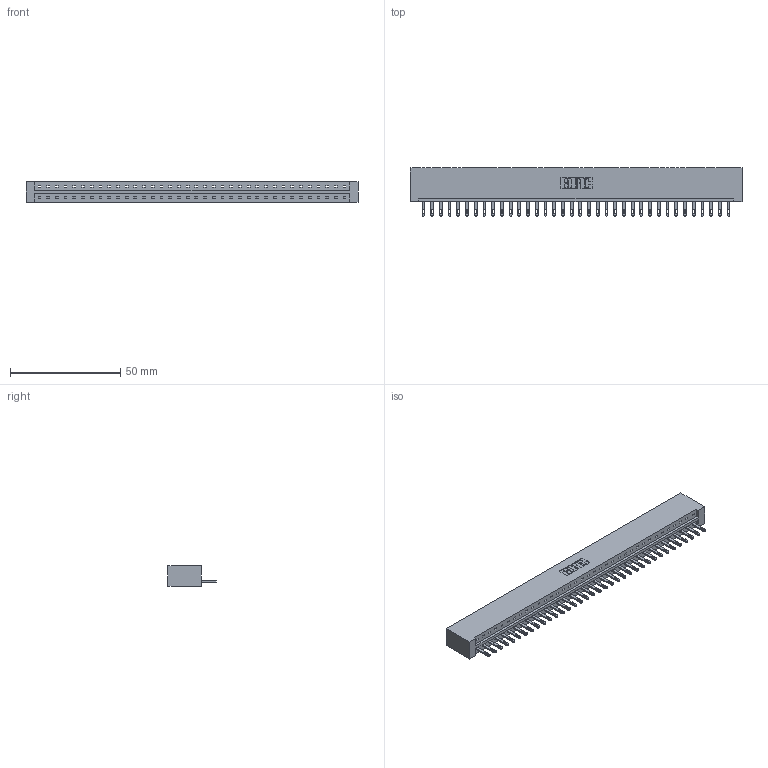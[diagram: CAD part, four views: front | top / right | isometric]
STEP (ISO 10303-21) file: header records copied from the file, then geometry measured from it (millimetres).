
FILE_DESCRIPTION (( 'STEP AP203' ), '1' );
FILE_NAME ('833-036-500-101.STEP', '2020-06-03T01:19:00', ( '' ), ( '' ), 'SwSTEP 2.0', 'SolidWorks 2020', '' );
FILE_SCHEMA (( 'CONFIG_CONTROL_DESIGN' ));
Length unit declared in the file: inch
Products named in the file (3): 833 Part_Lugless; 345-292-001_345-293-100; 833-036-500-101
Assembly tree (37 placements, depth 2):
  833-036-500-101
    833 Part_Lugless
    345-292-001_345-293-100  x36
Bounding box: 150.9 x 21.85 x 9.4 mm (x, y, z)
Volume: 15768.4 mm3; surface area: 17065.8 mm2
Topology: 37 solids, 37 shells, 2050 faces, 6335 edges, 4222 vertices
Faces by surface type: plane 1362, cylinder 688
Entity records: 22437 total; most frequent: CARTESIAN_POINT 3878, ORIENTED_EDGE 3850, DIRECTION 3277, EDGE_CURVE 1925, LINE 1801, VECTOR 1801, VERTEX_POINT 1282, AXIS2_PLACEMENT_3D 738
